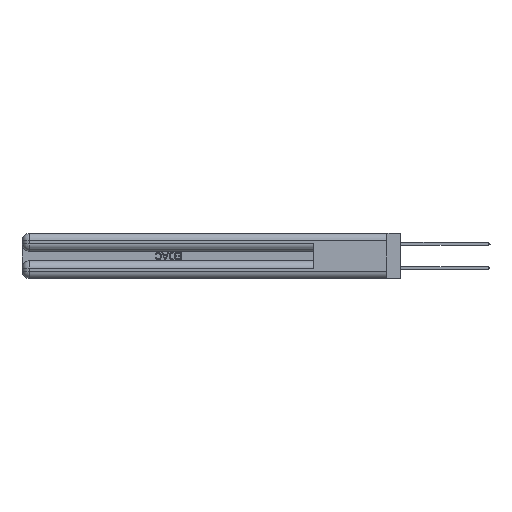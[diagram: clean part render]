
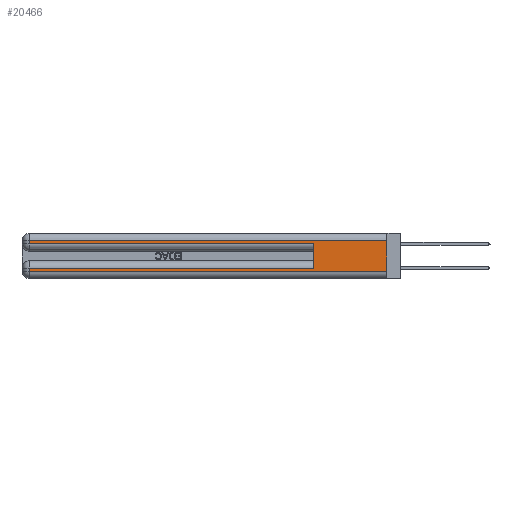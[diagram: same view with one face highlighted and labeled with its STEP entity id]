
A CAD part, left-side view. The second image highlights one B-rep face of the part: STEP entity #20466.
In plain terms, the highlighted planar face has unit normal (-1, 0, 0).
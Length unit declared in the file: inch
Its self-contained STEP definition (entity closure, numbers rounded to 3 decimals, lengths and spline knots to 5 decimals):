
#571 = AXIS2_PLACEMENT_3D ( 'NONE', #20671, #43592, #28423 ) ;
#1746 = EDGE_CURVE ( 'NONE', #24365, #16380, #2380, .T. ) ;
#1945 = LINE ( 'NONE', #21873, #41634 ) ;
#2380 = LINE ( 'NONE', #33499, #31855 ) ;
#2503 = CARTESIAN_POINT ( 'NONE',  ( 0., 0.6, 0.145 ) ) ;
#2512 = CARTESIAN_POINT ( 'NONE',  ( 0., 0., 0.31 ) ) ;
#2543 = FACE_OUTER_BOUND ( 'NONE', #36491, .T. ) ;
#3277 = CARTESIAN_POINT ( 'NONE',  ( 0., 2.94, 0.37 ) ) ;
#3689 = VECTOR ( 'NONE', #33280, 39.37008 ) ;
#4767 = EDGE_CURVE ( 'NONE', #44264, #25625, #1945, .T. ) ;
#5038 = DIRECTION ( 'NONE',  ( 0., -1., 0. ) ) ;
#5116 = ORIENTED_EDGE ( 'NONE', *, *, #8733, .F. ) ;
#6117 = CARTESIAN_POINT ( 'NONE',  ( 0., 2.94, 0.085 ) ) ;
#7161 = VECTOR ( 'NONE', #11632, 39.37008 ) ;
#8140 = DIRECTION ( 'NONE',  ( 0., 0., -1. ) ) ;
#8733 = EDGE_CURVE ( 'NONE', #25014, #23900, #18925, .T. ) ;
#8743 = VECTOR ( 'NONE', #42622, 39.37008 ) ;
#11632 = DIRECTION ( 'NONE',  ( 0., 1., 0. ) ) ;
#12495 = ORIENTED_EDGE ( 'NONE', *, *, #34601, .T. ) ;
#12717 = CARTESIAN_POINT ( 'NONE',  ( 0., 0., 0.06 ) ) ;
#14258 = ORIENTED_EDGE ( 'NONE', *, *, #1746, .T. ) ;
#15350 = CARTESIAN_POINT ( 'NONE',  ( 0., 0., 0.085 ) ) ;
#16380 = VERTEX_POINT ( 'NONE', #36220 ) ;
#17050 = CARTESIAN_POINT ( 'NONE',  ( 0., 0.6, 0.085 ) ) ;
#18460 = ORIENTED_EDGE ( 'NONE', *, *, #24096, .T. ) ;
#18925 = LINE ( 'NONE', #31182, #30390 ) ;
#19506 = VERTEX_POINT ( 'NONE', #38877 ) ;
#19805 = LINE ( 'NONE', #12717, #39107 ) ;
#20466 = ADVANCED_FACE ( 'NONE', ( #2543 ), #24532, .F. ) ;
#20671 = CARTESIAN_POINT ( 'NONE',  ( 0., 0., 0.37 ) ) ;
#21873 = CARTESIAN_POINT ( 'NONE',  ( 0., 0., 0.285 ) ) ;
#23900 = VERTEX_POINT ( 'NONE', #41611 ) ;
#24096 = EDGE_CURVE ( 'NONE', #25014, #19506, #38226, .T. ) ;
#24365 = VERTEX_POINT ( 'NONE', #6117 ) ;
#24532 = PLANE ( 'NONE',  #571 ) ;
#25014 = VERTEX_POINT ( 'NONE', #2512 ) ;
#25625 = VERTEX_POINT ( 'NONE', #29002 ) ;
#25756 = CARTESIAN_POINT ( 'NONE',  ( 0., 2.94, 0.285 ) ) ;
#26269 = ORIENTED_EDGE ( 'NONE', *, *, #41056, .T. ) ;
#26653 = VECTOR ( 'NONE', #37893, 39.37008 ) ;
#27708 = EDGE_CURVE ( 'NONE', #16380, #23900, #19805, .T. ) ;
#27846 = LINE ( 'NONE', #3277, #26653 ) ;
#28423 = DIRECTION ( 'NONE',  ( 0., 0., -1. ) ) ;
#28815 = LINE ( 'NONE', #15350, #7161 ) ;
#29002 = CARTESIAN_POINT ( 'NONE',  ( 0., 0.6, 0.285 ) ) ;
#29587 = DIRECTION ( 'NONE',  ( 0., 0., -1. ) ) ;
#30390 = VECTOR ( 'NONE', #8140, 39.37008 ) ;
#31182 = CARTESIAN_POINT ( 'NONE',  ( 0., 0., 0.37 ) ) ;
#31855 = VECTOR ( 'NONE', #29587, 39.37008 ) ;
#33280 = DIRECTION ( 'NONE',  ( 0., 0., 1. ) ) ;
#33499 = CARTESIAN_POINT ( 'NONE',  ( 0., 2.94, 0.37 ) ) ;
#33541 = DIRECTION ( 'NONE',  ( 0., -1., 0. ) ) ;
#34601 = EDGE_CURVE ( 'NONE', #19506, #44264, #27846, .T. ) ;
#36220 = CARTESIAN_POINT ( 'NONE',  ( 0., 2.94, 0.06 ) ) ;
#36276 = VERTEX_POINT ( 'NONE', #17050 ) ;
#36491 = EDGE_LOOP ( 'NONE', ( #5116, #18460, #12495, #44350, #48536, #26269, #14258, #48025 ) ) ;
#37893 = DIRECTION ( 'NONE',  ( 0., 0., -1. ) ) ;
#38226 = LINE ( 'NONE', #43121, #8743 ) ;
#38877 = CARTESIAN_POINT ( 'NONE',  ( 0., 2.94, 0.31 ) ) ;
#39107 = VECTOR ( 'NONE', #5038, 39.37008 ) ;
#39806 = EDGE_CURVE ( 'NONE', #36276, #25625, #44625, .T. ) ;
#41056 = EDGE_CURVE ( 'NONE', #36276, #24365, #28815, .T. ) ;
#41611 = CARTESIAN_POINT ( 'NONE',  ( 0., 0., 0.06 ) ) ;
#41634 = VECTOR ( 'NONE', #33541, 39.37008 ) ;
#42622 = DIRECTION ( 'NONE',  ( 0., 1., 0. ) ) ;
#43121 = CARTESIAN_POINT ( 'NONE',  ( 0., 0., 0.31 ) ) ;
#43592 = DIRECTION ( 'NONE',  ( 1., 0., 0. ) ) ;
#44264 = VERTEX_POINT ( 'NONE', #25756 ) ;
#44350 = ORIENTED_EDGE ( 'NONE', *, *, #4767, .T. ) ;
#44625 = LINE ( 'NONE', #2503, #3689 ) ;
#48025 = ORIENTED_EDGE ( 'NONE', *, *, #27708, .T. ) ;
#48536 = ORIENTED_EDGE ( 'NONE', *, *, #39806, .F. ) ;
